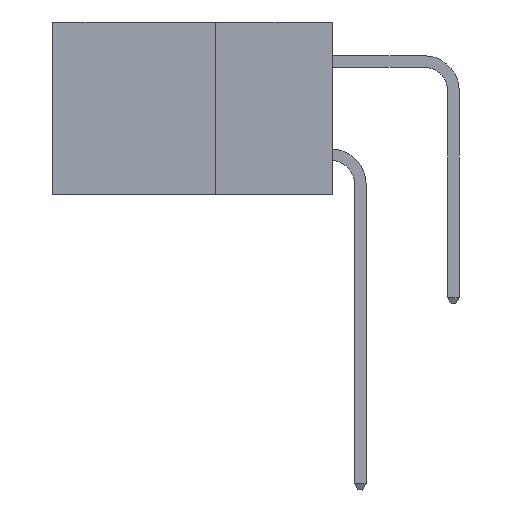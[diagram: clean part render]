
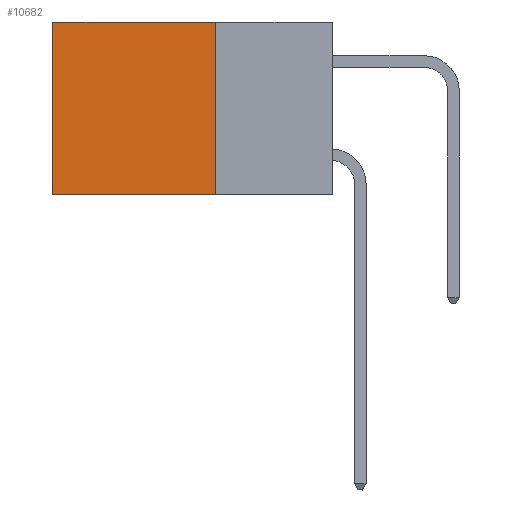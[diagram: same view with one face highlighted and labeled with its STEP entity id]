
A CAD part, left-side view. The second image highlights one B-rep face of the part: STEP entity #10682.
In plain terms, the highlighted planar face has unit normal (-1, 0, 0).
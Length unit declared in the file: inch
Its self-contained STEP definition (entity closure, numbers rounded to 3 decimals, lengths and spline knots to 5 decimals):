
#197 = EDGE_CURVE ( 'NONE', #15277, #1686, #3447, .T. ) ;
#1686 = VERTEX_POINT ( 'NONE', #14435 ) ;
#1820 = EDGE_CURVE ( 'NONE', #8483, #11126, #19427, .T. ) ;
#2656 = CARTESIAN_POINT ( 'NONE',  ( 0.298, 0.6, 0. ) ) ;
#2927 = DIRECTION ( 'NONE',  ( 0., 0., -1. ) ) ;
#3029 = CARTESIAN_POINT ( 'NONE',  ( 0.298, 0.25, 0. ) ) ;
#3447 = LINE ( 'NONE', #3029, #15677 ) ;
#3974 = EDGE_CURVE ( 'NONE', #15277, #8483, #7246, .T. ) ;
#4490 = DIRECTION ( 'NONE',  ( 0., 1., 0. ) ) ;
#6583 = EDGE_CURVE ( 'NONE', #1686, #11126, #12322, .T. ) ;
#7246 = LINE ( 'NONE', #13913, #15026 ) ;
#7485 = EDGE_LOOP ( 'NONE', ( #8774, #20093, #9105, #14556 ) ) ;
#7937 = VECTOR ( 'NONE', #4490, 39.37008 ) ;
#8483 = VERTEX_POINT ( 'NONE', #2656 ) ;
#8757 = FACE_OUTER_BOUND ( 'NONE', #7485, .T. ) ;
#8774 = ORIENTED_EDGE ( 'NONE', *, *, #1820, .T. ) ;
#8905 = CARTESIAN_POINT ( 'NONE',  ( 0.298, 0.25, -0.37 ) ) ;
#9105 = ORIENTED_EDGE ( 'NONE', *, *, #197, .F. ) ;
#9296 = CARTESIAN_POINT ( 'NONE',  ( 0.298, 0.25, 0. ) ) ;
#10682 = ADVANCED_FACE ( 'NONE', ( #8757 ), #19141, .F. ) ;
#10935 = DIRECTION ( 'NONE',  ( 0., 0., -1. ) ) ;
#11126 = VERTEX_POINT ( 'NONE', #20248 ) ;
#11276 = AXIS2_PLACEMENT_3D ( 'NONE', #9296, #20763, #10935 ) ;
#11293 = CARTESIAN_POINT ( 'NONE',  ( 0.298, 0.6, 0. ) ) ;
#12322 = LINE ( 'NONE', #8905, #7937 ) ;
#13913 = CARTESIAN_POINT ( 'NONE',  ( 0.298, 0.25, 0. ) ) ;
#14435 = CARTESIAN_POINT ( 'NONE',  ( 0.298, 0.25, -0.37 ) ) ;
#14540 = DIRECTION ( 'NONE',  ( 0., 1., 0. ) ) ;
#14556 = ORIENTED_EDGE ( 'NONE', *, *, #3974, .T. ) ;
#15026 = VECTOR ( 'NONE', #14540, 39.37008 ) ;
#15128 = VECTOR ( 'NONE', #16012, 39.37008 ) ;
#15277 = VERTEX_POINT ( 'NONE', #17771 ) ;
#15677 = VECTOR ( 'NONE', #2927, 39.37008 ) ;
#16012 = DIRECTION ( 'NONE',  ( 0., 0., -1. ) ) ;
#17771 = CARTESIAN_POINT ( 'NONE',  ( 0.298, 0.25, 0. ) ) ;
#19141 = PLANE ( 'NONE',  #11276 ) ;
#19427 = LINE ( 'NONE', #11293, #15128 ) ;
#20093 = ORIENTED_EDGE ( 'NONE', *, *, #6583, .F. ) ;
#20248 = CARTESIAN_POINT ( 'NONE',  ( 0.298, 0.6, -0.37 ) ) ;
#20763 = DIRECTION ( 'NONE',  ( 1., 0., 0. ) ) ;
